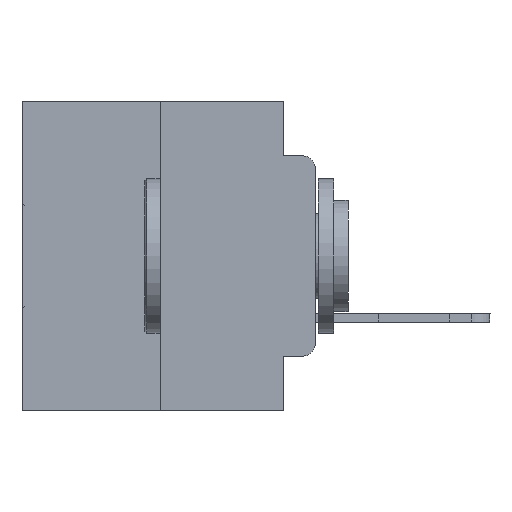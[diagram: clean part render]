
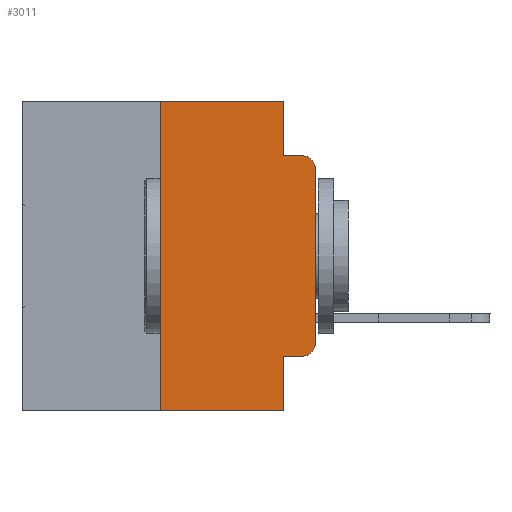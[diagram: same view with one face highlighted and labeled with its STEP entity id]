
A CAD part, left-side view. The second image highlights one B-rep face of the part: STEP entity #3011.
In plain terms, the highlighted planar face has unit normal (-1, 0, 0).
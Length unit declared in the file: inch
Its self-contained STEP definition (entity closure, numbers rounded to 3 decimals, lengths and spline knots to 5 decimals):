
#282 = CARTESIAN_POINT ( 'NONE',  ( 0., 0.473, 0. ) ) ;
#1284 = CARTESIAN_POINT ( 'NONE',  ( 0., 0.051, -0.0885 ) ) ;
#1661 = DIRECTION ( 'NONE',  ( 1., 0., 0. ) ) ;
#1841 = AXIS2_PLACEMENT_3D ( 'NONE', #18343, #25589, #30305 ) ;
#1994 = ORIENTED_EDGE ( 'NONE', *, *, #8769, .F. ) ;
#2474 = LINE ( 'NONE', #282, #23544 ) ;
#3011 = ADVANCED_FACE ( 'NONE', ( #18436 ), #25208, .F. ) ;
#3013 = EDGE_CURVE ( 'NONE', #26341, #20556, #18270, .T. ) ;
#3149 = CARTESIAN_POINT ( 'NONE',  ( 0., 0., -0.1085 ) ) ;
#3674 = ORIENTED_EDGE ( 'NONE', *, *, #6469, .F. ) ;
#3878 = DIRECTION ( 'NONE',  ( 0., 0., -1. ) ) ;
#3954 = LINE ( 'NONE', #21169, #25171 ) ;
#4558 = ORIENTED_EDGE ( 'NONE', *, *, #25824, .T. ) ;
#5199 = CARTESIAN_POINT ( 'NONE',  ( 0., 0.051, -0.4115 ) ) ;
#5782 = EDGE_CURVE ( 'NONE', #23787, #14184, #30149, .T. ) ;
#6008 = ORIENTED_EDGE ( 'NONE', *, *, #27525, .T. ) ;
#6469 = EDGE_CURVE ( 'NONE', #20863, #26736, #2474, .T. ) ;
#6822 = ORIENTED_EDGE ( 'NONE', *, *, #19506, .T. ) ;
#7050 = VECTOR ( 'NONE', #21597, 39.37008 ) ;
#8029 = CARTESIAN_POINT ( 'NONE',  ( 0., 0.051, -0.5 ) ) ;
#8056 = DIRECTION ( 'NONE',  ( 0., -1., 0. ) ) ;
#8769 = EDGE_CURVE ( 'NONE', #26736, #23261, #3954, .T. ) ;
#9128 = DIRECTION ( 'NONE',  ( 0., 0., -1. ) ) ;
#9378 = EDGE_CURVE ( 'NONE', #15479, #20863, #24111, .T. ) ;
#9868 = EDGE_CURVE ( 'NONE', #23261, #29448, #24078, .T. ) ;
#10200 = AXIS2_PLACEMENT_3D ( 'NONE', #25844, #14045, #9128 ) ;
#10712 = ORIENTED_EDGE ( 'NONE', *, *, #9378, .F. ) ;
#11949 = CARTESIAN_POINT ( 'NONE',  ( 0., 0.25, 0. ) ) ;
#12122 = DIRECTION ( 'NONE',  ( 0., -1., 0. ) ) ;
#12360 = LINE ( 'NONE', #27019, #27987 ) ;
#12671 = DIRECTION ( 'NONE',  ( 0., -1., 0. ) ) ;
#14045 = DIRECTION ( 'NONE',  ( -1., 0., 0. ) ) ;
#14184 = VERTEX_POINT ( 'NONE', #3149 ) ;
#14404 = EDGE_LOOP ( 'NONE', ( #26271, #6822, #25019, #1994, #3674, #10712, #20960, #19021, #6008, #4558 ) ) ;
#14510 = CARTESIAN_POINT ( 'NONE',  ( 0., 0.051, 0. ) ) ;
#14611 = CARTESIAN_POINT ( 'NONE',  ( 0., 0., -0.3915 ) ) ;
#15479 = VERTEX_POINT ( 'NONE', #16331 ) ;
#16331 = CARTESIAN_POINT ( 'NONE',  ( 0., 0.25, -0.5 ) ) ;
#16384 = EDGE_CURVE ( 'NONE', #15479, #20556, #12360, .T. ) ;
#17333 = VECTOR ( 'NONE', #27864, 39.37008 ) ;
#17962 = CARTESIAN_POINT ( 'NONE',  ( 0., 0.051, 0. ) ) ;
#18270 = LINE ( 'NONE', #17962, #17333 ) ;
#18343 = CARTESIAN_POINT ( 'NONE',  ( 0., 0.02, -0.3915 ) ) ;
#18436 = FACE_OUTER_BOUND ( 'NONE', #14404, .T. ) ;
#18808 = DIRECTION ( 'NONE',  ( 0., 0., -1. ) ) ;
#19021 = ORIENTED_EDGE ( 'NONE', *, *, #3013, .F. ) ;
#19049 = CARTESIAN_POINT ( 'NONE',  ( 0., 0.051, -0.0885 ) ) ;
#19506 = EDGE_CURVE ( 'NONE', #14184, #29448, #24805, .T. ) ;
#19997 = CARTESIAN_POINT ( 'NONE',  ( 0., 0.02, -0.4115 ) ) ;
#20556 = VERTEX_POINT ( 'NONE', #8029 ) ;
#20863 = VERTEX_POINT ( 'NONE', #11949 ) ;
#20960 = ORIENTED_EDGE ( 'NONE', *, *, #16384, .T. ) ;
#21169 = CARTESIAN_POINT ( 'NONE',  ( 0., 0.051, 0. ) ) ;
#21597 = DIRECTION ( 'NONE',  ( 0., 0., 1. ) ) ;
#23052 = CARTESIAN_POINT ( 'NONE',  ( 0., 0., 0. ) ) ;
#23261 = VERTEX_POINT ( 'NONE', #1284 ) ;
#23544 = VECTOR ( 'NONE', #12122, 39.37008 ) ;
#23787 = VERTEX_POINT ( 'NONE', #14611 ) ;
#24078 = LINE ( 'NONE', #19049, #29258 ) ;
#24111 = LINE ( 'NONE', #26478, #7050 ) ;
#24805 = CIRCLE ( 'NONE', #10200, 0.02 ) ;
#25019 = ORIENTED_EDGE ( 'NONE', *, *, #9868, .F. ) ;
#25171 = VECTOR ( 'NONE', #18808, 39.37008 ) ;
#25208 = PLANE ( 'NONE',  #28382 ) ;
#25260 = VERTEX_POINT ( 'NONE', #19997 ) ;
#25261 = DIRECTION ( 'NONE',  ( 0., 0., 1. ) ) ;
#25389 = CARTESIAN_POINT ( 'NONE',  ( 0., 0.051, -0.4115 ) ) ;
#25589 = DIRECTION ( 'NONE',  ( -1., 0., 0. ) ) ;
#25824 = EDGE_CURVE ( 'NONE', #25260, #23787, #29062, .T. ) ;
#25844 = CARTESIAN_POINT ( 'NONE',  ( 0., 0.02, -0.1085 ) ) ;
#26271 = ORIENTED_EDGE ( 'NONE', *, *, #5782, .T. ) ;
#26341 = VERTEX_POINT ( 'NONE', #25389 ) ;
#26478 = CARTESIAN_POINT ( 'NONE',  ( 0., 0.25, 0. ) ) ;
#26736 = VERTEX_POINT ( 'NONE', #14510 ) ;
#26820 = LINE ( 'NONE', #5199, #31177 ) ;
#27019 = CARTESIAN_POINT ( 'NONE',  ( 0., 0.473, -0.5 ) ) ;
#27525 = EDGE_CURVE ( 'NONE', #26341, #25260, #26820, .T. ) ;
#27864 = DIRECTION ( 'NONE',  ( 0., 0., -1. ) ) ;
#27961 = CARTESIAN_POINT ( 'NONE',  ( 0., 0.02, -0.0885 ) ) ;
#27987 = VECTOR ( 'NONE', #12671, 39.37008 ) ;
#28180 = CARTESIAN_POINT ( 'NONE',  ( 0., 0.473, 0. ) ) ;
#28382 = AXIS2_PLACEMENT_3D ( 'NONE', #28180, #1661, #3878 ) ;
#28652 = DIRECTION ( 'NONE',  ( 0., -1., 0. ) ) ;
#29062 = CIRCLE ( 'NONE', #1841, 0.02 ) ;
#29258 = VECTOR ( 'NONE', #28652, 39.37008 ) ;
#29448 = VERTEX_POINT ( 'NONE', #27961 ) ;
#29559 = VECTOR ( 'NONE', #25261, 39.37008 ) ;
#30149 = LINE ( 'NONE', #23052, #29559 ) ;
#30305 = DIRECTION ( 'NONE',  ( 0., 0., -1. ) ) ;
#31177 = VECTOR ( 'NONE', #8056, 39.37008 ) ;
